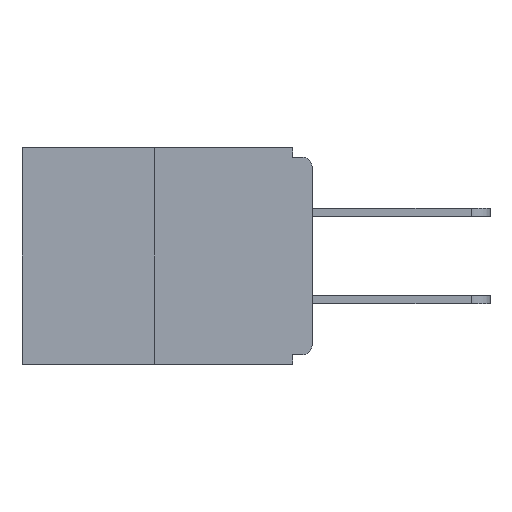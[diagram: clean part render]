
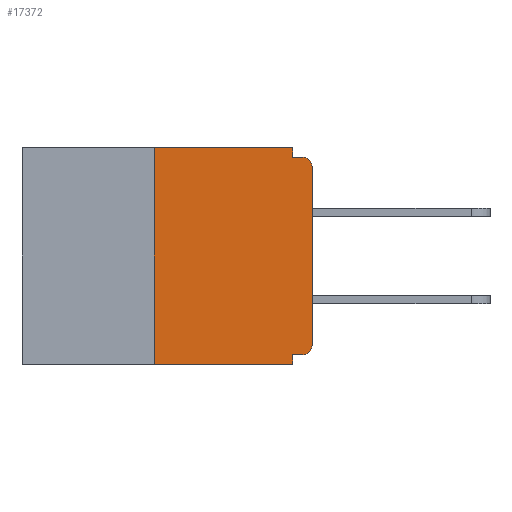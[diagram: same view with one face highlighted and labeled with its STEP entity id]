
A CAD part, left-side view. The second image highlights one B-rep face of the part: STEP entity #17372.
In plain terms, the highlighted planar face has unit normal (-1, 0, 0).
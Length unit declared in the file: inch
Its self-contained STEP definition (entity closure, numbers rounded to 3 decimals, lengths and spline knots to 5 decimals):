
#130 = DIRECTION ( 'NONE',  ( 0., 1., 0. ) ) ;
#310 = CARTESIAN_POINT ( 'NONE',  ( 0., 0., 0. ) ) ;
#533 = ORIENTED_EDGE ( 'NONE', *, *, #2731, .T. ) ;
#576 = VECTOR ( 'NONE', #16227, 39.37008 ) ;
#794 = CARTESIAN_POINT ( 'NONE',  ( 0., 0.015, -0.328 ) ) ;
#1127 = DIRECTION ( 'NONE',  ( -1., 0., 0. ) ) ;
#1984 = VERTEX_POINT ( 'NONE', #7137 ) ;
#2319 = ORIENTED_EDGE ( 'NONE', *, *, #16538, .F. ) ;
#2361 = FACE_OUTER_BOUND ( 'NONE', #2938, .T. ) ;
#2731 = EDGE_CURVE ( 'NONE', #16010, #8188, #10434, .T. ) ;
#2938 = EDGE_LOOP ( 'NONE', ( #5898, #16119, #13857, #2319, #6264, #533, #15528, #8144, #13890, #17464 ) ) ;
#3294 = VECTOR ( 'NONE', #130, 39.37008 ) ;
#3483 = LINE ( 'NONE', #13294, #15360 ) ;
#3584 = CARTESIAN_POINT ( 'NONE',  ( 0., 0.46, 0. ) ) ;
#4256 = VERTEX_POINT ( 'NONE', #17690 ) ;
#4258 = AXIS2_PLACEMENT_3D ( 'NONE', #13738, #17791, #14991 ) ;
#4383 = DIRECTION ( 'NONE',  ( 0., 0., 1. ) ) ;
#4755 = CARTESIAN_POINT ( 'NONE',  ( 0., 0.031, -0.343 ) ) ;
#5196 = LINE ( 'NONE', #9021, #5616 ) ;
#5292 = CARTESIAN_POINT ( 'NONE',  ( 0., 0.031, -0.328 ) ) ;
#5355 = DIRECTION ( 'NONE',  ( 0., 0., -1. ) ) ;
#5616 = VECTOR ( 'NONE', #14275, 39.37008 ) ;
#5898 = ORIENTED_EDGE ( 'NONE', *, *, #16567, .F. ) ;
#6076 = VERTEX_POINT ( 'NONE', #5292 ) ;
#6254 = LINE ( 'NONE', #3584, #7134 ) ;
#6264 = ORIENTED_EDGE ( 'NONE', *, *, #16160, .F. ) ;
#6329 = DIRECTION ( 'NONE',  ( 0., 0., -1. ) ) ;
#6690 = VECTOR ( 'NONE', #4383, 39.37008 ) ;
#6854 = LINE ( 'NONE', #17505, #14023 ) ;
#6933 = CARTESIAN_POINT ( 'NONE',  ( 0., 0., -0.328 ) ) ;
#7046 = DIRECTION ( 'NONE',  ( 0., 0., -1. ) ) ;
#7134 = VECTOR ( 'NONE', #14291, 39.37008 ) ;
#7137 = CARTESIAN_POINT ( 'NONE',  ( 0., 0.031, -0.015 ) ) ;
#7814 = CARTESIAN_POINT ( 'NONE',  ( 0., 0.015, -0.313 ) ) ;
#8144 = ORIENTED_EDGE ( 'NONE', *, *, #15823, .T. ) ;
#8188 = VERTEX_POINT ( 'NONE', #13113 ) ;
#9021 = CARTESIAN_POINT ( 'NONE',  ( 0., 0.031, 0. ) ) ;
#9268 = AXIS2_PLACEMENT_3D ( 'NONE', #7814, #10598, #6329 ) ;
#9384 = EDGE_CURVE ( 'NONE', #1984, #14939, #13479, .T. ) ;
#10215 = VERTEX_POINT ( 'NONE', #10453 ) ;
#10434 = CIRCLE ( 'NONE', #9268, 0.015 ) ;
#10453 = CARTESIAN_POINT ( 'NONE',  ( 0., 0.25, 0. ) ) ;
#10598 = DIRECTION ( 'NONE',  ( -1., 0., 0. ) ) ;
#10603 = VERTEX_POINT ( 'NONE', #14197 ) ;
#10657 = CIRCLE ( 'NONE', #17088, 0.015 ) ;
#10860 = LINE ( 'NONE', #6933, #3294 ) ;
#10879 = CARTESIAN_POINT ( 'NONE',  ( 0., 0.015, -0.03 ) ) ;
#11228 = EDGE_CURVE ( 'NONE', #10603, #1984, #5196, .T. ) ;
#11900 = EDGE_CURVE ( 'NONE', #4256, #13602, #6854, .T. ) ;
#12021 = VERTEX_POINT ( 'NONE', #17804 ) ;
#13113 = CARTESIAN_POINT ( 'NONE',  ( 0., 0., -0.313 ) ) ;
#13294 = CARTESIAN_POINT ( 'NONE',  ( 0., 0.031, -0.343 ) ) ;
#13336 = CARTESIAN_POINT ( 'NONE',  ( 0., 0., -0.015 ) ) ;
#13386 = DIRECTION ( 'NONE',  ( 0., -1., 0. ) ) ;
#13479 = LINE ( 'NONE', #13336, #576 ) ;
#13602 = VERTEX_POINT ( 'NONE', #4755 ) ;
#13617 = VECTOR ( 'NONE', #13916, 39.37008 ) ;
#13738 = CARTESIAN_POINT ( 'NONE',  ( 0., 0.46, 0. ) ) ;
#13857 = ORIENTED_EDGE ( 'NONE', *, *, #11900, .T. ) ;
#13890 = ORIENTED_EDGE ( 'NONE', *, *, #9384, .F. ) ;
#13916 = DIRECTION ( 'NONE',  ( 0., 0., 1. ) ) ;
#14023 = VECTOR ( 'NONE', #13386, 39.37008 ) ;
#14197 = CARTESIAN_POINT ( 'NONE',  ( 0., 0.031, 0. ) ) ;
#14275 = DIRECTION ( 'NONE',  ( 0., 0., -1. ) ) ;
#14291 = DIRECTION ( 'NONE',  ( 0., -1., 0. ) ) ;
#14939 = VERTEX_POINT ( 'NONE', #17064 ) ;
#14991 = DIRECTION ( 'NONE',  ( 0., 0., -1. ) ) ;
#15239 = PLANE ( 'NONE',  #4258 ) ;
#15358 = CARTESIAN_POINT ( 'NONE',  ( 0., 0.25, 0. ) ) ;
#15360 = VECTOR ( 'NONE', #7046, 39.37008 ) ;
#15528 = ORIENTED_EDGE ( 'NONE', *, *, #16742, .T. ) ;
#15823 = EDGE_CURVE ( 'NONE', #12021, #14939, #10657, .T. ) ;
#16010 = VERTEX_POINT ( 'NONE', #794 ) ;
#16119 = ORIENTED_EDGE ( 'NONE', *, *, #16717, .F. ) ;
#16160 = EDGE_CURVE ( 'NONE', #16010, #6076, #10860, .T. ) ;
#16227 = DIRECTION ( 'NONE',  ( 0., -1., 0. ) ) ;
#16538 = EDGE_CURVE ( 'NONE', #6076, #13602, #3483, .T. ) ;
#16567 = EDGE_CURVE ( 'NONE', #10215, #10603, #6254, .T. ) ;
#16717 = EDGE_CURVE ( 'NONE', #4256, #10215, #17310, .T. ) ;
#16742 = EDGE_CURVE ( 'NONE', #8188, #12021, #17533, .T. ) ;
#17064 = CARTESIAN_POINT ( 'NONE',  ( 0., 0.015, -0.015 ) ) ;
#17088 = AXIS2_PLACEMENT_3D ( 'NONE', #10879, #1127, #5355 ) ;
#17310 = LINE ( 'NONE', #15358, #6690 ) ;
#17372 = ADVANCED_FACE ( 'NONE', ( #2361 ), #15239, .F. ) ;
#17464 = ORIENTED_EDGE ( 'NONE', *, *, #11228, .F. ) ;
#17505 = CARTESIAN_POINT ( 'NONE',  ( 0., 0.46, -0.343 ) ) ;
#17533 = LINE ( 'NONE', #310, #13617 ) ;
#17690 = CARTESIAN_POINT ( 'NONE',  ( 0., 0.25, -0.343 ) ) ;
#17791 = DIRECTION ( 'NONE',  ( 1., 0., 0. ) ) ;
#17804 = CARTESIAN_POINT ( 'NONE',  ( 0., 0., -0.03 ) ) ;
